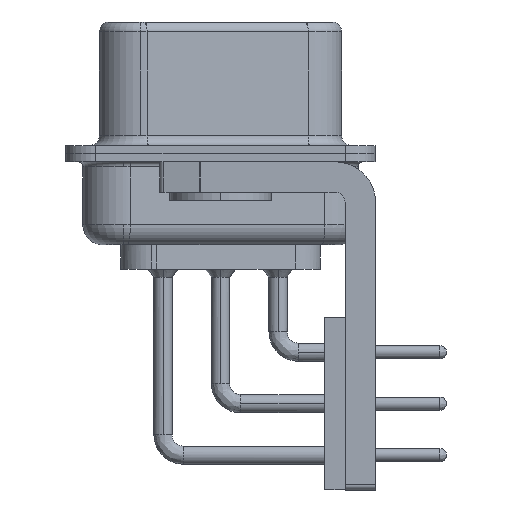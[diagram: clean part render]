
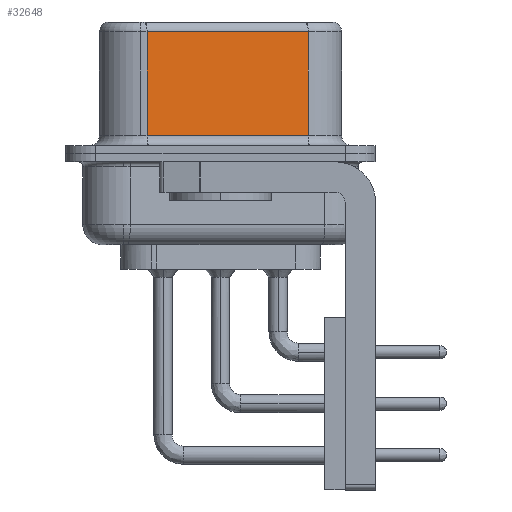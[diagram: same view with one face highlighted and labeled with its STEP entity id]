
A CAD part, left-side view. The second image highlights one B-rep face of the part: STEP entity #32648.
In plain terms, the highlighted planar face has unit normal (-0.985, -0.174, 0).
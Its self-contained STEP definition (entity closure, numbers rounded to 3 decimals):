
#1734 = ORIENTED_EDGE ( 'NONE', *, *, #6782, .F. ) ;
#2382 = CARTESIAN_POINT ( 'NONE',  ( 5.132, -4.322, 6.52 ) ) ;
#5948 = DIRECTION ( 'NONE',  ( 0.174, -0.985, 0. ) ) ;
#6782 = EDGE_CURVE ( 'NONE', #36681, #21458, #35372, .T. ) ;
#7919 = LINE ( 'NONE', #37088, #15437 ) ;
#9195 = CARTESIAN_POINT ( 'NONE',  ( 5.132, -4.322, 0.9 ) ) ;
#9866 = FACE_OUTER_BOUND ( 'NONE', #24279, .T. ) ;
#11041 = ORIENTED_EDGE ( 'NONE', *, *, #28445, .T. ) ;
#12786 = CARTESIAN_POINT ( 'NONE',  ( 3.73, 3.628, 6.52 ) ) ;
#13899 = DIRECTION ( 'NONE',  ( -0.174, 0.985, 0. ) ) ;
#14120 = VECTOR ( 'NONE', #5948, 1000. ) ;
#15437 = VECTOR ( 'NONE', #24064, 1000. ) ;
#16931 = LINE ( 'NONE', #12786, #34266 ) ;
#19639 = ORIENTED_EDGE ( 'NONE', *, *, #31722, .T. ) ;
#21352 = CARTESIAN_POINT ( 'NONE',  ( 5.132, -4.322, 6.02 ) ) ;
#21458 = VERTEX_POINT ( 'NONE', #24255 ) ;
#23530 = CARTESIAN_POINT ( 'NONE',  ( 5.132, -4.322, 6.52 ) ) ;
#24064 = DIRECTION ( 'NONE',  ( -0.174, 0.985, 0. ) ) ;
#24189 = EDGE_CURVE ( 'NONE', #25445, #21458, #31434, .T. ) ;
#24255 = CARTESIAN_POINT ( 'NONE',  ( 5.132, -4.322, 0.9 ) ) ;
#24279 = EDGE_LOOP ( 'NONE', ( #1734, #19639, #11041, #31853 ) ) ;
#24598 = VECTOR ( 'NONE', #37996, 1000. ) ;
#25445 = VERTEX_POINT ( 'NONE', #28932 ) ;
#27822 = AXIS2_PLACEMENT_3D ( 'NONE', #23530, #33402, #13899 ) ;
#28445 = EDGE_CURVE ( 'NONE', #29927, #25445, #16931, .T. ) ;
#28932 = CARTESIAN_POINT ( 'NONE',  ( 3.73, 3.628, 0.9 ) ) ;
#29927 = VERTEX_POINT ( 'NONE', #31951 ) ;
#30107 = PLANE ( 'NONE',  #27822 ) ;
#31434 = LINE ( 'NONE', #9195, #14120 ) ;
#31722 = EDGE_CURVE ( 'NONE', #36681, #29927, #7919, .T. ) ;
#31853 = ORIENTED_EDGE ( 'NONE', *, *, #24189, .T. ) ;
#31951 = CARTESIAN_POINT ( 'NONE',  ( 3.73, 3.628, 6.02 ) ) ;
#32648 = ADVANCED_FACE ( 'NONE', ( #9866 ), #30107, .F. ) ;
#33402 = DIRECTION ( 'NONE',  ( 0.985, 0.174, 0. ) ) ;
#34266 = VECTOR ( 'NONE', #35568, 1000. ) ;
#35372 = LINE ( 'NONE', #2382, #24598 ) ;
#35568 = DIRECTION ( 'NONE',  ( 0., 0., -1. ) ) ;
#36681 = VERTEX_POINT ( 'NONE', #21352 ) ;
#37088 = CARTESIAN_POINT ( 'NONE',  ( 5.132, -4.322, 6.02 ) ) ;
#37996 = DIRECTION ( 'NONE',  ( 0., 0., -1. ) ) ;
